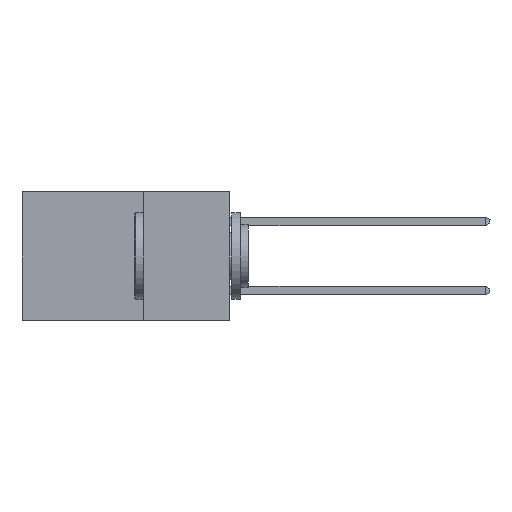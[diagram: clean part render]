
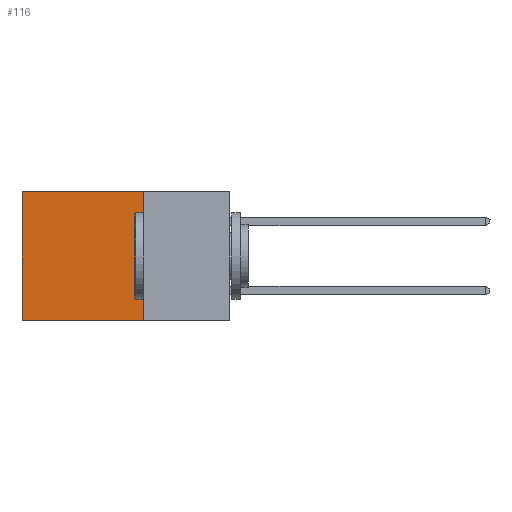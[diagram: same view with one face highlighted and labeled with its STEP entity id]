
A CAD part, left-side view. The second image highlights one B-rep face of the part: STEP entity #116.
In plain terms, the highlighted planar face has unit normal (-1, 0, 0).
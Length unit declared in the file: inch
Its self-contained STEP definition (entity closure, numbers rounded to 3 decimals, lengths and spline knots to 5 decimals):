
#116 = ADVANCED_FACE ( 'NONE', ( #1537 ), #10890, .F. ) ;
#858 = LINE ( 'NONE', #3762, #1928 ) ;
#1537 = FACE_OUTER_BOUND ( 'NONE', #8265, .T. ) ;
#1928 = VECTOR ( 'NONE', #10104, 39.37008 ) ;
#2001 = EDGE_CURVE ( 'NONE', #14483, #11421, #7564, .T. ) ;
#2226 = VERTEX_POINT ( 'NONE', #7140 ) ;
#2806 = VECTOR ( 'NONE', #17496, 39.37008 ) ;
#2825 = DIRECTION ( 'NONE',  ( 0., 0., -1. ) ) ;
#3762 = CARTESIAN_POINT ( 'NONE',  ( 0.2615, 0.25, 0. ) ) ;
#4431 = DIRECTION ( 'NONE',  ( 0., 1., 0. ) ) ;
#4585 = CARTESIAN_POINT ( 'NONE',  ( 0.2615, 0.25, -0.37 ) ) ;
#4626 = CARTESIAN_POINT ( 'NONE',  ( 0.2615, 0.25, -0.37 ) ) ;
#5242 = LINE ( 'NONE', #11399, #2806 ) ;
#5649 = ORIENTED_EDGE ( 'NONE', *, *, #9022, .T. ) ;
#6602 = VERTEX_POINT ( 'NONE', #18403 ) ;
#7140 = CARTESIAN_POINT ( 'NONE',  ( 0.2615, 0.25, 0. ) ) ;
#7564 = LINE ( 'NONE', #4626, #19691 ) ;
#7776 = CARTESIAN_POINT ( 'NONE',  ( 0.2615, 0.25, -0.37 ) ) ;
#8265 = EDGE_LOOP ( 'NONE', ( #5649, #17006, #9225, #8535 ) ) ;
#8535 = ORIENTED_EDGE ( 'NONE', *, *, #18330, .T. ) ;
#8548 = AXIS2_PLACEMENT_3D ( 'NONE', #7776, #13697, #18212 ) ;
#8959 = LINE ( 'NONE', #10861, #15300 ) ;
#9022 = EDGE_CURVE ( 'NONE', #6602, #11421, #8959, .T. ) ;
#9225 = ORIENTED_EDGE ( 'NONE', *, *, #11392, .F. ) ;
#10104 = DIRECTION ( 'NONE',  ( 0., 1., 0. ) ) ;
#10861 = CARTESIAN_POINT ( 'NONE',  ( 0.2615, 0.6, -0.37 ) ) ;
#10890 = PLANE ( 'NONE',  #8548 ) ;
#11392 = EDGE_CURVE ( 'NONE', #2226, #14483, #5242, .T. ) ;
#11399 = CARTESIAN_POINT ( 'NONE',  ( 0.2615, 0.25, -0.37 ) ) ;
#11421 = VERTEX_POINT ( 'NONE', #12008 ) ;
#12008 = CARTESIAN_POINT ( 'NONE',  ( 0.2615, 0.6, -0.37 ) ) ;
#13697 = DIRECTION ( 'NONE',  ( 1., 0., 0. ) ) ;
#14483 = VERTEX_POINT ( 'NONE', #4585 ) ;
#15300 = VECTOR ( 'NONE', #2825, 39.37008 ) ;
#17006 = ORIENTED_EDGE ( 'NONE', *, *, #2001, .F. ) ;
#17496 = DIRECTION ( 'NONE',  ( 0., 0., -1. ) ) ;
#18212 = DIRECTION ( 'NONE',  ( 0., 0., -1. ) ) ;
#18330 = EDGE_CURVE ( 'NONE', #2226, #6602, #858, .T. ) ;
#18403 = CARTESIAN_POINT ( 'NONE',  ( 0.2615, 0.6, 0. ) ) ;
#19691 = VECTOR ( 'NONE', #4431, 39.37008 ) ;
